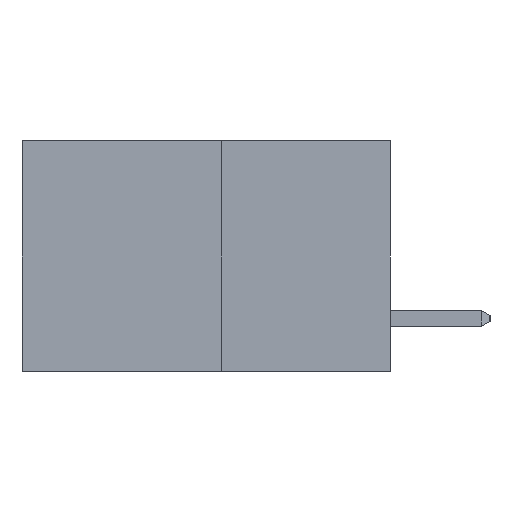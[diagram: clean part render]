
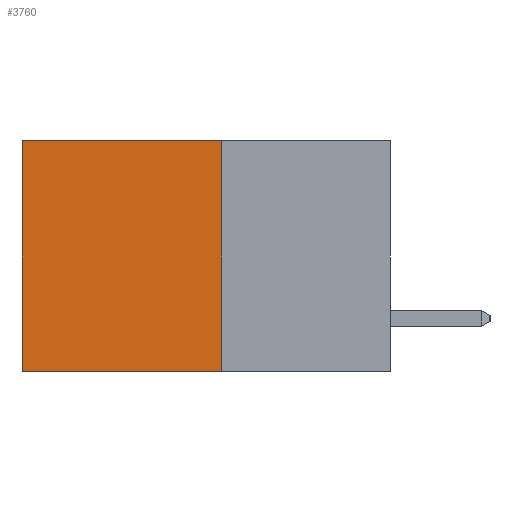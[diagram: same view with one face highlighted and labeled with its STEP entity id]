
A CAD part, left-side view. The second image highlights one B-rep face of the part: STEP entity #3760.
In plain terms, the highlighted planar face has unit normal (-1, 0, 0).
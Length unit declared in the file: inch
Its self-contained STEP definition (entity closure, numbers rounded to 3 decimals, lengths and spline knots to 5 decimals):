
#593 = VECTOR ( 'NONE', #4185, 39.37008 ) ;
#1320 = ORIENTED_EDGE ( 'NONE', *, *, #2903, .F. ) ;
#1566 = CARTESIAN_POINT ( 'NONE',  ( 0.277, 0.27, 0. ) ) ;
#1667 = LINE ( 'NONE', #5790, #7783 ) ;
#1965 = FACE_OUTER_BOUND ( 'NONE', #11878, .T. ) ;
#2670 = LINE ( 'NONE', #2881, #11718 ) ;
#2777 = VERTEX_POINT ( 'NONE', #1566 ) ;
#2881 = CARTESIAN_POINT ( 'NONE',  ( 0.277, 0.59, -0.37 ) ) ;
#2903 = EDGE_CURVE ( 'NONE', #4716, #8237, #8119, .T. ) ;
#3760 = ADVANCED_FACE ( 'NONE', ( #1965 ), #10928, .F. ) ;
#4051 = VERTEX_POINT ( 'NONE', #8647 ) ;
#4185 = DIRECTION ( 'NONE',  ( 0., 0., -1. ) ) ;
#4225 = ORIENTED_EDGE ( 'NONE', *, *, #13650, .T. ) ;
#4436 = AXIS2_PLACEMENT_3D ( 'NONE', #10951, #8933, #8899 ) ;
#4716 = VERTEX_POINT ( 'NONE', #5084 ) ;
#4887 = VECTOR ( 'NONE', #13176, 39.37008 ) ;
#5084 = CARTESIAN_POINT ( 'NONE',  ( 0.277, 0.27, -0.37 ) ) ;
#5664 = DIRECTION ( 'NONE',  ( 0., 1., 0. ) ) ;
#5674 = CARTESIAN_POINT ( 'NONE',  ( 0.277, 0.27, -0.37 ) ) ;
#5790 = CARTESIAN_POINT ( 'NONE',  ( 0.277, 0.27, 0. ) ) ;
#7520 = LINE ( 'NONE', #10294, #593 ) ;
#7783 = VECTOR ( 'NONE', #5664, 39.37008 ) ;
#8119 = LINE ( 'NONE', #5674, #4887 ) ;
#8216 = ORIENTED_EDGE ( 'NONE', *, *, #8649, .T. ) ;
#8237 = VERTEX_POINT ( 'NONE', #14478 ) ;
#8647 = CARTESIAN_POINT ( 'NONE',  ( 0.277, 0.59, 0. ) ) ;
#8649 = EDGE_CURVE ( 'NONE', #2777, #4051, #1667, .T. ) ;
#8899 = DIRECTION ( 'NONE',  ( 0., 0., -1. ) ) ;
#8933 = DIRECTION ( 'NONE',  ( 1., 0., 0. ) ) ;
#10294 = CARTESIAN_POINT ( 'NONE',  ( 0.277, 0.27, -0.37 ) ) ;
#10704 = EDGE_CURVE ( 'NONE', #2777, #4716, #7520, .T. ) ;
#10928 = PLANE ( 'NONE',  #4436 ) ;
#10951 = CARTESIAN_POINT ( 'NONE',  ( 0.277, 0.27, -0.37 ) ) ;
#11718 = VECTOR ( 'NONE', #12774, 39.37008 ) ;
#11878 = EDGE_LOOP ( 'NONE', ( #4225, #1320, #15535, #8216 ) ) ;
#12774 = DIRECTION ( 'NONE',  ( 0., 0., -1. ) ) ;
#13176 = DIRECTION ( 'NONE',  ( 0., 1., 0. ) ) ;
#13650 = EDGE_CURVE ( 'NONE', #4051, #8237, #2670, .T. ) ;
#14478 = CARTESIAN_POINT ( 'NONE',  ( 0.277, 0.59, -0.37 ) ) ;
#15535 = ORIENTED_EDGE ( 'NONE', *, *, #10704, .F. ) ;
